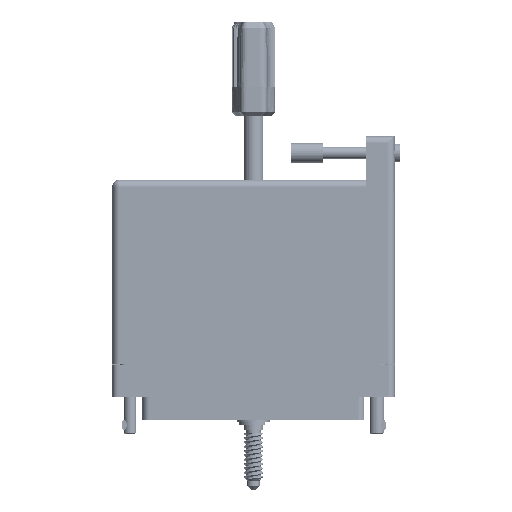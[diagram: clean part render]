
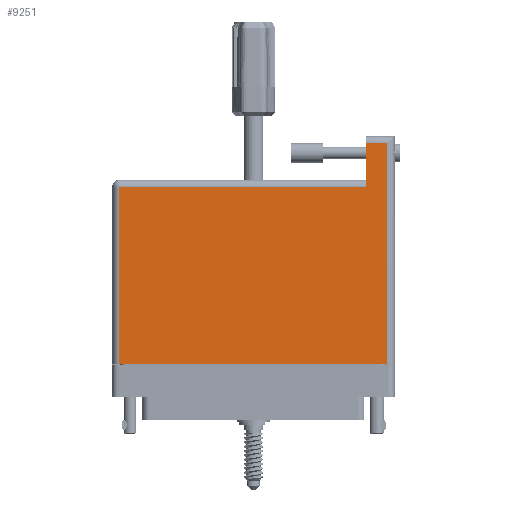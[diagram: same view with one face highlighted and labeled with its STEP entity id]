
A CAD part, front view. The second image highlights one B-rep face of the part: STEP entity #9251.
In plain terms, the highlighted face is planar.
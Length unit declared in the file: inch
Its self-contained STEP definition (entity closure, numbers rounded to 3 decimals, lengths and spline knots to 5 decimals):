
#5231 = CARTESIAN_POINT ( 'NONE',  ( 1.079, 1.605, 0.617 ) ) ;
#5639 = VERTEX_POINT ( 'NONE', #5231 ) ;
#9251 = ADVANCED_FACE ( 'NONE', ( #44601 ), #19072, .F. ) ;
#9740 = CARTESIAN_POINT ( 'NONE',  ( 1.289, 2.095, 0.617 ) ) ;
#12541 = CARTESIAN_POINT ( 'NONE',  ( -1.359, 1.675, 0.617 ) ) ;
#12587 = CARTESIAN_POINT ( 'NONE',  ( -1.289, -0.1, 0.617 ) ) ;
#12969 = EDGE_CURVE ( 'NONE', #5639, #14955, #77003, .T. ) ;
#13671 = DIRECTION ( 'NONE',  ( -1., 0., 0. ) ) ;
#14955 = VERTEX_POINT ( 'NONE', #67054 ) ;
#15630 = CARTESIAN_POINT ( 'NONE',  ( 1.079, 2.095, 0.617 ) ) ;
#17348 = CARTESIAN_POINT ( 'NONE',  ( -1.359, 2.025, 0.617 ) ) ;
#19072 = PLANE ( 'NONE',  #49235 ) ;
#22259 = LINE ( 'NONE', #17348, #84363 ) ;
#22695 = VERTEX_POINT ( 'NONE', #30197 ) ;
#24124 = LINE ( 'NONE', #47254, #60411 ) ;
#30197 = CARTESIAN_POINT ( 'NONE',  ( 1.289, 2.025, 0.617 ) ) ;
#33566 = DIRECTION ( 'NONE',  ( 0., 0., -1. ) ) ;
#33902 = DIRECTION ( 'NONE',  ( -1., 0., 0. ) ) ;
#34270 = VECTOR ( 'NONE', #67953, 39.37008 ) ;
#35081 = VECTOR ( 'NONE', #84988, 39.37008 ) ;
#37881 = VERTEX_POINT ( 'NONE', #71542 ) ;
#40060 = LINE ( 'NONE', #15630, #34270 ) ;
#43155 = CARTESIAN_POINT ( 'NONE',  ( -1.359, 1.605, 0.617 ) ) ;
#44601 = FACE_OUTER_BOUND ( 'NONE', #79573, .T. ) ;
#45416 = VERTEX_POINT ( 'NONE', #12587 ) ;
#47254 = CARTESIAN_POINT ( 'NONE',  ( -1.359, -0.1, 0.617 ) ) ;
#48786 = EDGE_CURVE ( 'NONE', #45416, #37881, #24124, .T. ) ;
#49235 = AXIS2_PLACEMENT_3D ( 'NONE', #12541, #33566, #33902 ) ;
#54370 = DIRECTION ( 'NONE',  ( 1., 0., 0. ) ) ;
#56265 = VERTEX_POINT ( 'NONE', #83203 ) ;
#60411 = VECTOR ( 'NONE', #54370, 39.37008 ) ;
#60904 = EDGE_CURVE ( 'NONE', #37881, #22695, #92361, .T. ) ;
#63400 = EDGE_CURVE ( 'NONE', #14955, #45416, #65182, .T. ) ;
#65182 = LINE ( 'NONE', #81139, #87403 ) ;
#67018 = DIRECTION ( 'NONE',  ( 0., -1., 0. ) ) ;
#67054 = CARTESIAN_POINT ( 'NONE',  ( -1.289, 1.605, 0.617 ) ) ;
#67953 = DIRECTION ( 'NONE',  ( 0., -1., 0. ) ) ;
#69304 = ORIENTED_EDGE ( 'NONE', *, *, #86627, .T. ) ;
#71542 = CARTESIAN_POINT ( 'NONE',  ( 1.289, -0.1, 0.617 ) ) ;
#73655 = ORIENTED_EDGE ( 'NONE', *, *, #80027, .T. ) ;
#75805 = ORIENTED_EDGE ( 'NONE', *, *, #48786, .T. ) ;
#77003 = LINE ( 'NONE', #43155, #82771 ) ;
#79573 = EDGE_LOOP ( 'NONE', ( #94715, #87347, #75805, #93464, #73655, #69304 ) ) ;
#80027 = EDGE_CURVE ( 'NONE', #22695, #56265, #22259, .T. ) ;
#81139 = CARTESIAN_POINT ( 'NONE',  ( -1.289, -0.1, 0.617 ) ) ;
#82771 = VECTOR ( 'NONE', #13671, 39.37008 ) ;
#83203 = CARTESIAN_POINT ( 'NONE',  ( 1.079, 2.025, 0.617 ) ) ;
#84363 = VECTOR ( 'NONE', #92249, 39.37008 ) ;
#84988 = DIRECTION ( 'NONE',  ( 0., 1., 0. ) ) ;
#86627 = EDGE_CURVE ( 'NONE', #56265, #5639, #40060, .T. ) ;
#87347 = ORIENTED_EDGE ( 'NONE', *, *, #63400, .T. ) ;
#87403 = VECTOR ( 'NONE', #67018, 39.37008 ) ;
#92249 = DIRECTION ( 'NONE',  ( -1., 0., 0. ) ) ;
#92361 = LINE ( 'NONE', #9740, #35081 ) ;
#93464 = ORIENTED_EDGE ( 'NONE', *, *, #60904, .T. ) ;
#94715 = ORIENTED_EDGE ( 'NONE', *, *, #12969, .T. ) ;
